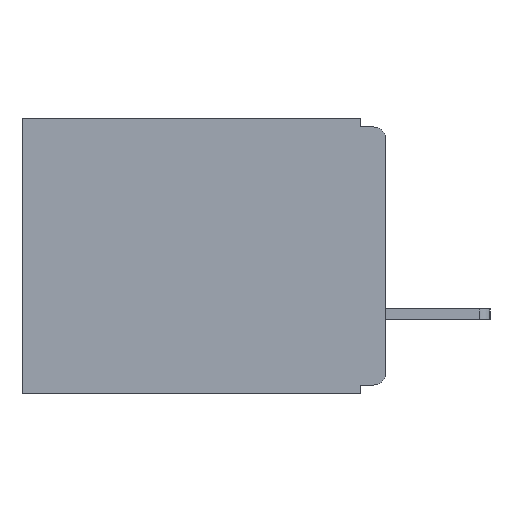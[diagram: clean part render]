
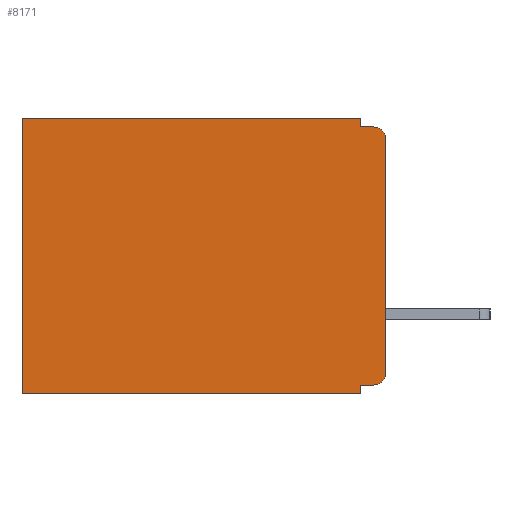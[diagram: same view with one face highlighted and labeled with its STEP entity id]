
A CAD part, left-side view. The second image highlights one B-rep face of the part: STEP entity #8171.
In plain terms, the highlighted planar face has unit normal (-1, 0, 0).
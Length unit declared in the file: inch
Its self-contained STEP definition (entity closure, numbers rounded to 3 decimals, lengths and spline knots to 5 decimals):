
#13 = DIRECTION ( 'NONE',  ( 0., 0., -1. ) ) ;
#1233 = AXIS2_PLACEMENT_3D ( 'NONE', #12146, #12089, #12071 ) ;
#1249 = CARTESIAN_POINT ( 'NONE',  ( 0.3, 0.031, 0. ) ) ;
#1708 = CARTESIAN_POINT ( 'NONE',  ( 0.3, 0.015, -0.32 ) ) ;
#1731 = EDGE_CURVE ( 'NONE', #6548, #2336, #10868, .T. ) ;
#1950 = VERTEX_POINT ( 'NONE', #7649 ) ;
#1981 = CARTESIAN_POINT ( 'NONE',  ( 0.3, 0.437, -0.33 ) ) ;
#2334 = CARTESIAN_POINT ( 'NONE',  ( 0.3, 0.015, -0.01 ) ) ;
#2336 = VERTEX_POINT ( 'NONE', #3262 ) ;
#2758 = DIRECTION ( 'NONE',  ( 0., -1., 0. ) ) ;
#2817 = LINE ( 'NONE', #15392, #15234 ) ;
#2994 = CARTESIAN_POINT ( 'NONE',  ( 0.3, 0.031, -0.01 ) ) ;
#3013 = LINE ( 'NONE', #9889, #15388 ) ;
#3184 = CIRCLE ( 'NONE', #6723, 0.015 ) ;
#3262 = CARTESIAN_POINT ( 'NONE',  ( 0.3, 0.437, -0.33 ) ) ;
#3392 = EDGE_CURVE ( 'NONE', #1950, #9287, #2817, .T. ) ;
#3554 = EDGE_CURVE ( 'NONE', #12236, #3991, #3013, .T. ) ;
#3690 = EDGE_CURVE ( 'NONE', #4642, #13070, #10963, .T. ) ;
#3765 = EDGE_CURVE ( 'NONE', #1950, #3991, #3184, .T. ) ;
#3861 = EDGE_CURVE ( 'NONE', #4642, #9287, #11140, .T. ) ;
#3991 = VERTEX_POINT ( 'NONE', #2334 ) ;
#4035 = VECTOR ( 'NONE', #12301, 39.37008 ) ;
#4266 = DIRECTION ( 'NONE',  ( 0., 0., -1. ) ) ;
#4642 = VERTEX_POINT ( 'NONE', #1708 ) ;
#4726 = CARTESIAN_POINT ( 'NONE',  ( 0.3, 0., -0.305 ) ) ;
#4797 = EDGE_LOOP ( 'NONE', ( #14643, #6089, #15090, #15231, #15254, #15662, #6312, #13401, #7312, #5656 ) ) ;
#5293 = EDGE_CURVE ( 'NONE', #6812, #2336, #10626, .T. ) ;
#5319 = CARTESIAN_POINT ( 'NONE',  ( 0.3, 0.015, -0.025 ) ) ;
#5553 = DIRECTION ( 'NONE',  ( -1., 0., 0. ) ) ;
#5564 = EDGE_CURVE ( 'NONE', #9812, #12236, #11341, .T. ) ;
#5567 = EDGE_CURVE ( 'NONE', #13070, #6812, #8166, .T. ) ;
#5656 = ORIENTED_EDGE ( 'NONE', *, *, #3861, .T. ) ;
#5716 = CARTESIAN_POINT ( 'NONE',  ( 0.3, 0., -0.33 ) ) ;
#5857 = FACE_OUTER_BOUND ( 'NONE', #4797, .T. ) ;
#6089 = ORIENTED_EDGE ( 'NONE', *, *, #3765, .T. ) ;
#6204 = LINE ( 'NONE', #8895, #15572 ) ;
#6312 = ORIENTED_EDGE ( 'NONE', *, *, #5293, .F. ) ;
#6508 = DIRECTION ( 'NONE',  ( 0., 1., 0. ) ) ;
#6548 = VERTEX_POINT ( 'NONE', #7940 ) ;
#6723 = AXIS2_PLACEMENT_3D ( 'NONE', #5319, #5553, #8928 ) ;
#6812 = VERTEX_POINT ( 'NONE', #12852 ) ;
#7265 = VECTOR ( 'NONE', #13, 39.37008 ) ;
#7312 = ORIENTED_EDGE ( 'NONE', *, *, #3690, .F. ) ;
#7325 = DIRECTION ( 'NONE',  ( 0., 0., -1. ) ) ;
#7562 = DIRECTION ( 'NONE',  ( -1., 0., 0. ) ) ;
#7649 = CARTESIAN_POINT ( 'NONE',  ( 0.3, 0., -0.025 ) ) ;
#7786 = VECTOR ( 'NONE', #11000, 39.37008 ) ;
#7856 = CARTESIAN_POINT ( 'NONE',  ( 0.3, 0., -0.32 ) ) ;
#7940 = CARTESIAN_POINT ( 'NONE',  ( 0.3, 0.437, 0. ) ) ;
#8166 = LINE ( 'NONE', #11120, #7786 ) ;
#8171 = ADVANCED_FACE ( 'NONE', ( #5857 ), #12183, .F. ) ;
#8895 = CARTESIAN_POINT ( 'NONE',  ( 0.3, 0., 0. ) ) ;
#8928 = DIRECTION ( 'NONE',  ( 0., 0., -1. ) ) ;
#9287 = VERTEX_POINT ( 'NONE', #4726 ) ;
#9812 = VERTEX_POINT ( 'NONE', #1249 ) ;
#9889 = CARTESIAN_POINT ( 'NONE',  ( 0.3, 0., -0.01 ) ) ;
#10592 = VECTOR ( 'NONE', #6508, 39.37008 ) ;
#10626 = LINE ( 'NONE', #5716, #4035 ) ;
#10868 = LINE ( 'NONE', #1981, #7265 ) ;
#10963 = LINE ( 'NONE', #7856, #10592 ) ;
#11000 = DIRECTION ( 'NONE',  ( 0., 0., -1. ) ) ;
#11120 = CARTESIAN_POINT ( 'NONE',  ( 0.3, 0.031, -0.33 ) ) ;
#11140 = CIRCLE ( 'NONE', #13099, 0.015 ) ;
#11328 = CARTESIAN_POINT ( 'NONE',  ( 0.3, 0.031, 0. ) ) ;
#11341 = LINE ( 'NONE', #11328, #14014 ) ;
#11349 = CARTESIAN_POINT ( 'NONE',  ( 0.3, 0.015, -0.305 ) ) ;
#11657 = DIRECTION ( 'NONE',  ( 0., 0., -1. ) ) ;
#12071 = DIRECTION ( 'NONE',  ( 0., 0., -1. ) ) ;
#12089 = DIRECTION ( 'NONE',  ( 1., 0., 0. ) ) ;
#12146 = CARTESIAN_POINT ( 'NONE',  ( 0.3, 0., -0.33 ) ) ;
#12183 = PLANE ( 'NONE',  #1233 ) ;
#12236 = VERTEX_POINT ( 'NONE', #2994 ) ;
#12301 = DIRECTION ( 'NONE',  ( 0., 1., 0. ) ) ;
#12852 = CARTESIAN_POINT ( 'NONE',  ( 0.3, 0.031, -0.33 ) ) ;
#13070 = VERTEX_POINT ( 'NONE', #14080 ) ;
#13099 = AXIS2_PLACEMENT_3D ( 'NONE', #11349, #7562, #7325 ) ;
#13401 = ORIENTED_EDGE ( 'NONE', *, *, #5567, .F. ) ;
#14014 = VECTOR ( 'NONE', #11657, 39.37008 ) ;
#14080 = CARTESIAN_POINT ( 'NONE',  ( 0.3, 0.031, -0.32 ) ) ;
#14546 = EDGE_CURVE ( 'NONE', #9812, #6548, #6204, .T. ) ;
#14643 = ORIENTED_EDGE ( 'NONE', *, *, #3392, .F. ) ;
#15090 = ORIENTED_EDGE ( 'NONE', *, *, #3554, .F. ) ;
#15231 = ORIENTED_EDGE ( 'NONE', *, *, #5564, .F. ) ;
#15234 = VECTOR ( 'NONE', #4266, 39.37008 ) ;
#15254 = ORIENTED_EDGE ( 'NONE', *, *, #14546, .T. ) ;
#15388 = VECTOR ( 'NONE', #2758, 39.37008 ) ;
#15392 = CARTESIAN_POINT ( 'NONE',  ( 0.3, 0., -0.33 ) ) ;
#15572 = VECTOR ( 'NONE', #15746, 39.37008 ) ;
#15662 = ORIENTED_EDGE ( 'NONE', *, *, #1731, .T. ) ;
#15746 = DIRECTION ( 'NONE',  ( 0., 1., 0. ) ) ;
